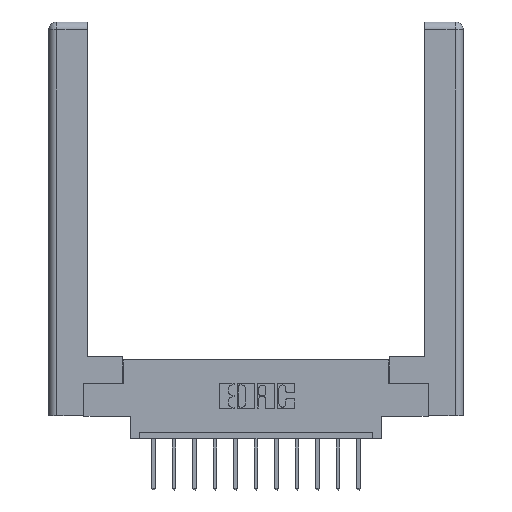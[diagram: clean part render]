
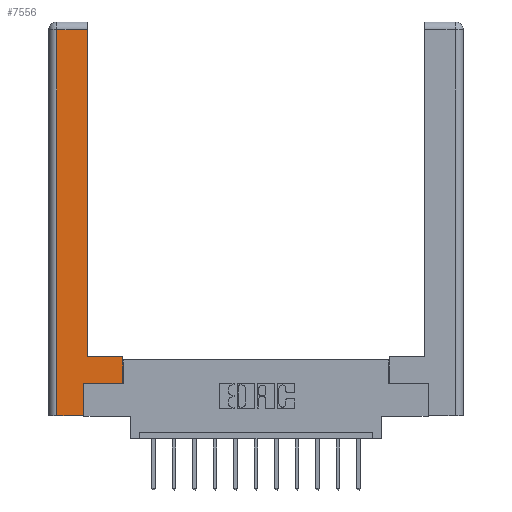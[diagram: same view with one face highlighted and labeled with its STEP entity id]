
A CAD part, top view. The second image highlights one B-rep face of the part: STEP entity #7556.
In plain terms, the highlighted planar face has unit normal (0, 0, 1).
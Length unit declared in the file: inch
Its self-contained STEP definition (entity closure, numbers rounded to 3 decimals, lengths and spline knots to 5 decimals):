
#37 = ORIENTED_EDGE ( 'NONE', *, *, #10101, .T. ) ;
#111 = DIRECTION ( 'NONE',  ( 0., -1., 0. ) ) ;
#277 = VECTOR ( 'NONE', #111, 39.37008 ) ;
#298 = CARTESIAN_POINT ( 'NONE',  ( 0.295, 0.45, 0. ) ) ;
#302 = EDGE_CURVE ( 'NONE', #11047, #1870, #12212, .T. ) ;
#313 = CARTESIAN_POINT ( 'NONE',  ( 0.265, 0.245, 0. ) ) ;
#466 = LINE ( 'NONE', #6494, #14214 ) ;
#866 = DIRECTION ( 'NONE',  ( -1., 0., 0. ) ) ;
#1028 = CARTESIAN_POINT ( 'NONE',  ( 0.295, 0.45, 0. ) ) ;
#1142 = LINE ( 'NONE', #8285, #6938 ) ;
#1335 = DIRECTION ( 'NONE',  ( 0., 1., 0. ) ) ;
#1544 = ORIENTED_EDGE ( 'NONE', *, *, #3334, .T. ) ;
#1743 = ORIENTED_EDGE ( 'NONE', *, *, #9093, .T. ) ;
#1870 = VERTEX_POINT ( 'NONE', #3824 ) ;
#2274 = VECTOR ( 'NONE', #866, 39.37008 ) ;
#2793 = DIRECTION ( 'NONE',  ( 1., 0., 0. ) ) ;
#2804 = ORIENTED_EDGE ( 'NONE', *, *, #8634, .T. ) ;
#3187 = VECTOR ( 'NONE', #8717, 39.37008 ) ;
#3334 = EDGE_CURVE ( 'NONE', #13941, #4335, #466, .T. ) ;
#3449 = CARTESIAN_POINT ( 'NONE',  ( 0.0615, 0., 0. ) ) ;
#3810 = DIRECTION ( 'NONE',  ( -1., 0., 0. ) ) ;
#3824 = CARTESIAN_POINT ( 'NONE',  ( 0.295, 2.94, 0. ) ) ;
#4093 = FACE_OUTER_BOUND ( 'NONE', #6622, .T. ) ;
#4200 = LINE ( 'NONE', #1028, #7661 ) ;
#4235 = CARTESIAN_POINT ( 'NONE',  ( 0.0615, 2.94, 0. ) ) ;
#4335 = VERTEX_POINT ( 'NONE', #11380 ) ;
#4354 = VECTOR ( 'NONE', #6956, 39.37008 ) ;
#4588 = CARTESIAN_POINT ( 'NONE',  ( 0.265, 0.245, 0. ) ) ;
#4699 = CARTESIAN_POINT ( 'NONE',  ( 0.0615, 0., 0. ) ) ;
#4718 = LINE ( 'NONE', #4588, #4354 ) ;
#4735 = AXIS2_PLACEMENT_3D ( 'NONE', #10547, #9449, #3810 ) ;
#5657 = DIRECTION ( 'NONE',  ( -1., 0., 0. ) ) ;
#5697 = LINE ( 'NONE', #4699, #277 ) ;
#5782 = ORIENTED_EDGE ( 'NONE', *, *, #9946, .T. ) ;
#5863 = VERTEX_POINT ( 'NONE', #313 ) ;
#6036 = PLANE ( 'NONE',  #4735 ) ;
#6126 = VERTEX_POINT ( 'NONE', #6442 ) ;
#6442 = CARTESIAN_POINT ( 'NONE',  ( 0.565, 0.45, 0. ) ) ;
#6494 = CARTESIAN_POINT ( 'NONE',  ( 0.265, 0., 0. ) ) ;
#6622 = EDGE_LOOP ( 'NONE', ( #13936, #1743, #2804, #1544, #6967, #12713, #37, #5782 ) ) ;
#6929 = EDGE_CURVE ( 'NONE', #5863, #9241, #7935, .T. ) ;
#6938 = VECTOR ( 'NONE', #1335, 39.37008 ) ;
#6954 = VERTEX_POINT ( 'NONE', #13993 ) ;
#6956 = DIRECTION ( 'NONE',  ( 0., 1., 0. ) ) ;
#6967 = ORIENTED_EDGE ( 'NONE', *, *, #10749, .T. ) ;
#7556 = ADVANCED_FACE ( 'NONE', ( #4093 ), #6036, .F. ) ;
#7661 = VECTOR ( 'NONE', #5657, 39.37008 ) ;
#7935 = LINE ( 'NONE', #13002, #10840 ) ;
#7999 = CARTESIAN_POINT ( 'NONE',  ( 0.565, 0.245, 0. ) ) ;
#8285 = CARTESIAN_POINT ( 'NONE',  ( 0.565, 0.45, 0. ) ) ;
#8410 = LINE ( 'NONE', #4235, #2274 ) ;
#8634 = EDGE_CURVE ( 'NONE', #6954, #13941, #5697, .T. ) ;
#8717 = DIRECTION ( 'NONE',  ( 0., 1., 0. ) ) ;
#9093 = EDGE_CURVE ( 'NONE', #1870, #6954, #8410, .T. ) ;
#9241 = VERTEX_POINT ( 'NONE', #7999 ) ;
#9449 = DIRECTION ( 'NONE',  ( 0., 0., -1. ) ) ;
#9946 = EDGE_CURVE ( 'NONE', #6126, #11047, #4200, .T. ) ;
#10101 = EDGE_CURVE ( 'NONE', #9241, #6126, #1142, .T. ) ;
#10547 = CARTESIAN_POINT ( 'NONE',  ( 0., 0., 0. ) ) ;
#10749 = EDGE_CURVE ( 'NONE', #4335, #5863, #4718, .T. ) ;
#10840 = VECTOR ( 'NONE', #2793, 39.37008 ) ;
#11047 = VERTEX_POINT ( 'NONE', #298 ) ;
#11380 = CARTESIAN_POINT ( 'NONE',  ( 0.265, 0., 0. ) ) ;
#12181 = CARTESIAN_POINT ( 'NONE',  ( 0.295, 3., 0. ) ) ;
#12212 = LINE ( 'NONE', #12181, #3187 ) ;
#12713 = ORIENTED_EDGE ( 'NONE', *, *, #6929, .T. ) ;
#13002 = CARTESIAN_POINT ( 'NONE',  ( 0.565, 0.245, 0. ) ) ;
#13936 = ORIENTED_EDGE ( 'NONE', *, *, #302, .T. ) ;
#13941 = VERTEX_POINT ( 'NONE', #3449 ) ;
#13993 = CARTESIAN_POINT ( 'NONE',  ( 0.0615, 2.94, 0. ) ) ;
#14214 = VECTOR ( 'NONE', #14728, 39.37008 ) ;
#14728 = DIRECTION ( 'NONE',  ( 1., 0., 0. ) ) ;
